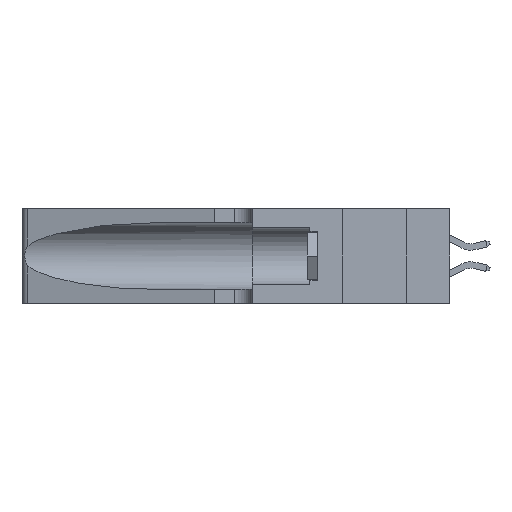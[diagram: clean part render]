
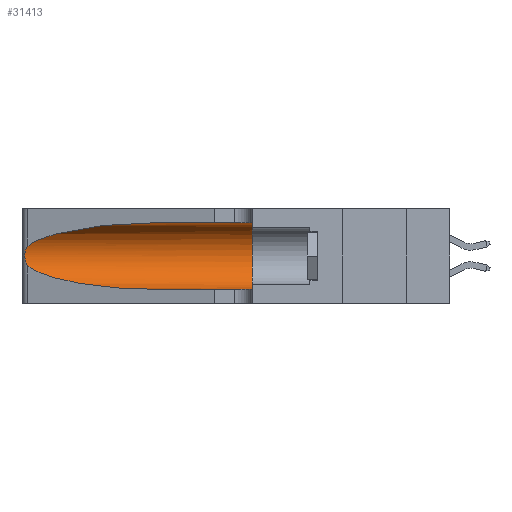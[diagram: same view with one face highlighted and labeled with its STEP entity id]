
A CAD part, left-side view. The second image highlights one B-rep face of the part: STEP entity #31413.
In plain terms, the highlighted cylindrical face has radius 3.308 mm (diameter 6.617 mm), a partial arc.
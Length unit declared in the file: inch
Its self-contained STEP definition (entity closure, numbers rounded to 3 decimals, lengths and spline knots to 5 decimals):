
#34 = CARTESIAN_POINT ( 'NONE',  ( 0.26018, 1.23835, 0.19895 ) ) ;
#282 = DIRECTION ( 'NONE',  ( 0., -1., 0. ) ) ;
#721 = ORIENTED_EDGE ( 'NONE', *, *, #18413, .T. ) ;
#914 = VERTEX_POINT ( 'NONE', #12960 ) ;
#1112 = DIRECTION ( 'NONE',  ( 0., 1., 0. ) ) ;
#1283 = CARTESIAN_POINT ( 'NONE',  ( 0.25487, 1.22718, 0.14631 ) ) ;
#1617 = VERTEX_POINT ( 'NONE', #25542 ) ;
#2385 = CARTESIAN_POINT ( 'NONE',  ( 0.2373, 1.15595, 0.28018 ) ) ;
#2646 = CARTESIAN_POINT ( 'NONE',  ( 0.26075, 1.23896, 0.178 ) ) ;
#3772 = VECTOR ( 'NONE', #282, 39.37008 ) ;
#3871 = CARTESIAN_POINT ( 'NONE',  ( 0.18966, 0.96281, 0.05475 ) ) ;
#4579 = CARTESIAN_POINT ( 'NONE',  ( 0.1305, 0.72297, 0.05475 ) ) ;
#4896 = ORIENTED_EDGE ( 'NONE', *, *, #15414, .F. ) ;
#5257 = CARTESIAN_POINT ( 'NONE',  ( 0.25856, 1.23593, 0.16098 ) ) ;
#5317 = ORIENTED_EDGE ( 'NONE', *, *, #30989, .F. ) ;
#7061 = CYLINDRICAL_SURFACE ( 'NONE', #19080, 0.13025 ) ;
#7229 = LINE ( 'NONE', #15699, #13260 ) ;
#7358 = B_SPLINE_CURVE_WITH_KNOTS ( 'NONE', 3,
 ( #7725, #30379, #12885, #30476, #15429, #34, #17992, #2646, #20550, #5257, #23067, #7851, #25606, #10451 ),
 .UNSPECIFIED., .F., .F.,
 ( 4, 2, 2, 2, 2, 2, 4 ),
 ( 0., 0.00027, 0.00053, 0.00107, 0.0016, 0.00187, 0.00214 ),
 .UNSPECIFIED. ) ;
#7679 = VERTEX_POINT ( 'NONE', #19643 ) ;
#7725 = CARTESIAN_POINT ( 'NONE',  ( 0.25487, 1.22718, 0.22369 ) ) ;
#7851 = CARTESIAN_POINT ( 'NONE',  ( 0.25639, 1.23186, 0.15144 ) ) ;
#10172 = AXIS2_PLACEMENT_3D ( 'NONE', #16446, #1112, #19047 ) ;
#10451 = CARTESIAN_POINT ( 'NONE',  ( 0.25487, 1.22718, 0.14631 ) ) ;
#10586 = VERTEX_POINT ( 'NONE', #25389 ) ;
#10602 = EDGE_CURVE ( 'NONE', #10586, #32684, #7358, .T. ) ;
#11663 = VERTEX_POINT ( 'NONE', #4579 ) ;
#12885 = CARTESIAN_POINT ( 'NONE',  ( 0.25639, 1.23184, 0.21858 ) ) ;
#12960 = CARTESIAN_POINT ( 'NONE',  ( 0.1305, 0.35, 0.31525 ) ) ;
#13022 = ORIENTED_EDGE ( 'NONE', *, *, #21950, .T. ) ;
#13260 = VECTOR ( 'NONE', #15812, 39.37008 ) ;
#15177 = CARTESIAN_POINT ( 'NONE',  ( 0.18966, 0.96281, 0.31525 ) ) ;
#15414 = EDGE_CURVE ( 'NONE', #914, #7679, #21502, .T. ) ;
#15429 = CARTESIAN_POINT ( 'NONE',  ( 0.25854, 1.2359, 0.20912 ) ) ;
#15699 = CARTESIAN_POINT ( 'NONE',  ( 0.1305, 1.61858, 0.31525 ) ) ;
#15812 = DIRECTION ( 'NONE',  ( 0., -1., 0. ) ) ;
#16446 = CARTESIAN_POINT ( 'NONE',  ( 0.1305, 0.35, 0.185 ) ) ;
#17366 = LINE ( 'NONE', #18231, #3772 ) ;
#17446 = DIRECTION ( 'NONE',  ( 0., 0., -1. ) ) ;
#17992 = CARTESIAN_POINT ( 'NONE',  ( 0.26075, 1.23896, 0.19203 ) ) ;
#18231 = CARTESIAN_POINT ( 'NONE',  ( 0.1305, 1.61858, 0.05475 ) ) ;
#18413 = EDGE_CURVE ( 'NONE', #1617, #10586, #28474, .T. ) ;
#19047 = DIRECTION ( 'NONE',  ( 0., 0., 1. ) ) ;
#19080 = AXIS2_PLACEMENT_3D ( 'NONE', #32489, #29979, #17446 ) ;
#19206 = CARTESIAN_POINT ( 'NONE',  ( 0.2373, 1.15595, 0.08982 ) ) ;
#19288 = EDGE_LOOP ( 'NONE', ( #721, #30611, #32832, #13022, #4896, #5317 ) ) ;
#19643 = CARTESIAN_POINT ( 'NONE',  ( 0.1305, 0.35, 0.05475 ) ) ;
#20178 = CARTESIAN_POINT ( 'NONE',  ( 0.1305, 0.72297, 0.31525 ) ) ;
#20238 =( BOUNDED_CURVE ( )  B_SPLINE_CURVE ( 3, ( #1283, #19206, #3871, #21742 ),
 .UNSPECIFIED., .F., .F. ) 
 B_SPLINE_CURVE_WITH_KNOTS ( ( 4, 4 ),
 ( 3.44316, 4.71239 ),
 .UNSPECIFIED. ) 
 CURVE ( )  GEOMETRIC_REPRESENTATION_ITEM ( )  RATIONAL_B_SPLINE_CURVE ( ( 1., 0.87, 0.87, 1. ) ) 
 REPRESENTATION_ITEM ( '' )  );
#20263 = CARTESIAN_POINT ( 'NONE',  ( 0.25487, 1.22718, 0.14631 ) ) ;
#20287 = CARTESIAN_POINT ( 'NONE',  ( 0.25487, 1.22718, 0.22369 ) ) ;
#20550 = CARTESIAN_POINT ( 'NONE',  ( 0.26017, 1.23833, 0.17102 ) ) ;
#20637 = FACE_OUTER_BOUND ( 'NONE', #19288, .T. ) ;
#21502 = CIRCLE ( 'NONE', #10172, 0.13025 ) ;
#21742 = CARTESIAN_POINT ( 'NONE',  ( 0.1305, 0.72297, 0.05475 ) ) ;
#21950 = EDGE_CURVE ( 'NONE', #11663, #7679, #17366, .T. ) ;
#23067 = CARTESIAN_POINT ( 'NONE',  ( 0.25789, 1.23486, 0.15765 ) ) ;
#25389 = CARTESIAN_POINT ( 'NONE',  ( 0.25487, 1.22718, 0.22369 ) ) ;
#25542 = CARTESIAN_POINT ( 'NONE',  ( 0.1305, 0.72297, 0.31525 ) ) ;
#25606 = CARTESIAN_POINT ( 'NONE',  ( 0.25555, 1.22993, 0.14849 ) ) ;
#28474 =( BOUNDED_CURVE ( )  B_SPLINE_CURVE ( 3, ( #20178, #15177, #2385, #20287 ),
 .UNSPECIFIED., .F., .F. ) 
 B_SPLINE_CURVE_WITH_KNOTS ( ( 4, 4 ),
 ( 1.5708, 2.84003 ),
 .UNSPECIFIED. ) 
 CURVE ( )  GEOMETRIC_REPRESENTATION_ITEM ( )  RATIONAL_B_SPLINE_CURVE ( ( 1., 0.87, 0.87, 1. ) ) 
 REPRESENTATION_ITEM ( '' )  );
#29979 = DIRECTION ( 'NONE',  ( 0., -1., 0. ) ) ;
#30379 = CARTESIAN_POINT ( 'NONE',  ( 0.25555, 1.22994, 0.2215 ) ) ;
#30476 = CARTESIAN_POINT ( 'NONE',  ( 0.25787, 1.23484, 0.2124 ) ) ;
#30611 = ORIENTED_EDGE ( 'NONE', *, *, #10602, .T. ) ;
#30989 = EDGE_CURVE ( 'NONE', #1617, #914, #7229, .T. ) ;
#31413 = ADVANCED_FACE ( 'NONE', ( #20637 ), #7061, .F. ) ;
#32489 = CARTESIAN_POINT ( 'NONE',  ( 0.1305, 1.61858, 0.185 ) ) ;
#32544 = EDGE_CURVE ( 'NONE', #32684, #11663, #20238, .T. ) ;
#32684 = VERTEX_POINT ( 'NONE', #20263 ) ;
#32832 = ORIENTED_EDGE ( 'NONE', *, *, #32544, .T. ) ;
